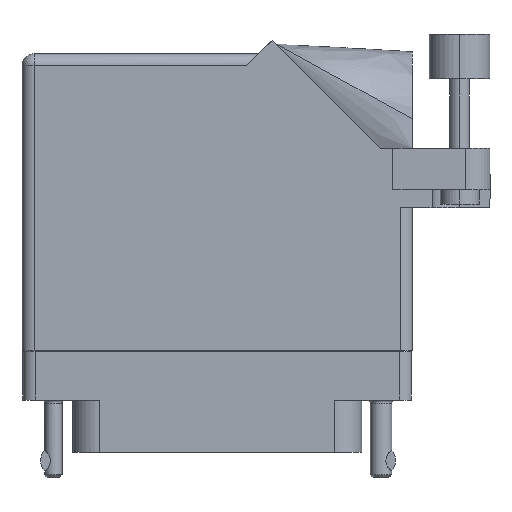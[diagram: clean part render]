
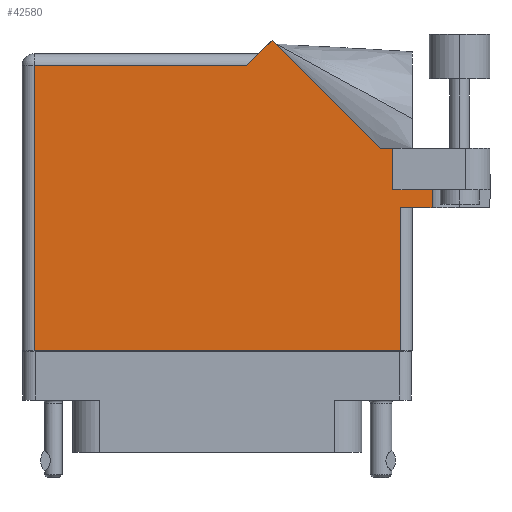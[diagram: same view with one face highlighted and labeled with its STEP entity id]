
A CAD part, front view. The second image highlights one B-rep face of the part: STEP entity #42580.
In plain terms, the highlighted face is planar.
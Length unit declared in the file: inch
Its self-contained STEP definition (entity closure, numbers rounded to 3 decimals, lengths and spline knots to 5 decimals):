
#213 = DIRECTION ( 'NONE',  ( 1., 0., 0. ) ) ;
#391 = CARTESIAN_POINT ( 'NONE',  ( -0.943, -0.1, 0.455 ) ) ;
#471 = PLANE ( 'NONE',  #19270 ) ;
#1316 = DIRECTION ( 'NONE',  ( 0., 1., 0. ) ) ;
#1674 = VECTOR ( 'NONE', #46622, 39.37008 ) ;
#4321 = CARTESIAN_POINT ( 'NONE',  ( -1.005, -0.1, 0.455 ) ) ;
#4349 = DIRECTION ( 'NONE',  ( 1., 0., 0. ) ) ;
#4591 = VERTEX_POINT ( 'NONE', #47811 ) ;
#5573 = DIRECTION ( 'NONE',  ( 1., 0., 0. ) ) ;
#5835 = CARTESIAN_POINT ( 'NONE',  ( 0.905, 0.731, 0.455 ) ) ;
#6892 = LINE ( 'NONE', #45167, #42203 ) ;
#7204 = EDGE_CURVE ( 'NONE', #48685, #36561, #42917, .T. ) ;
#8289 = CARTESIAN_POINT ( 'NONE',  ( -1.005, 1.43, 0.455 ) ) ;
#8791 = CARTESIAN_POINT ( 'NONE',  ( 0.943, 0.637, 0.455 ) ) ;
#9611 = LINE ( 'NONE', #45680, #19108 ) ;
#10578 = ORIENTED_EDGE ( 'NONE', *, *, #26713, .T. ) ;
#11178 = VECTOR ( 'NONE', #5573, 39.37008 ) ;
#11192 = VERTEX_POINT ( 'NONE', #36400 ) ;
#11431 = DIRECTION ( 'NONE',  ( -0.707, -0.707, 0. ) ) ;
#11445 = VERTEX_POINT ( 'NONE', #33540 ) ;
#11779 = CARTESIAN_POINT ( 'NONE',  ( 0.943, 0.637, 0.455 ) ) ;
#11818 = ORIENTED_EDGE ( 'NONE', *, *, #48078, .T. ) ;
#11912 = LINE ( 'NONE', #46286, #1674 ) ;
#11988 = VERTEX_POINT ( 'NONE', #46523 ) ;
#12066 = FACE_OUTER_BOUND ( 'NONE', #29427, .T. ) ;
#13126 = VECTOR ( 'NONE', #25380, 39.37008 ) ;
#14388 = LINE ( 'NONE', #33651, #33549 ) ;
#14573 = DIRECTION ( 'NONE',  ( 0., 1., 0. ) ) ;
#15288 = CARTESIAN_POINT ( 'NONE',  ( 0.83942, 0.944, 0.455 ) ) ;
#16756 = CARTESIAN_POINT ( 'NONE',  ( 1.1065, 0.637, 0.455 ) ) ;
#17214 = CARTESIAN_POINT ( 'NONE',  ( 1.005, 0.637, 0.455 ) ) ;
#17432 = LINE ( 'NONE', #8791, #44462 ) ;
#18132 = DIRECTION ( 'NONE',  ( -1., 0., 0. ) ) ;
#18425 = ORIENTED_EDGE ( 'NONE', *, *, #28230, .T. ) ;
#18794 = DIRECTION ( 'NONE',  ( -1., 0., 0. ) ) ;
#19108 = VECTOR ( 'NONE', #18794, 39.37008 ) ;
#19270 = AXIS2_PLACEMENT_3D ( 'NONE', #8289, #19598, #35013 ) ;
#19598 = DIRECTION ( 'NONE',  ( 0., 0., -1. ) ) ;
#20357 = EDGE_CURVE ( 'NONE', #48685, #4591, #14388, .T. ) ;
#20387 = LINE ( 'NONE', #48424, #45028 ) ;
#22706 = VECTOR ( 'NONE', #213, 39.37008 ) ;
#22811 = VERTEX_POINT ( 'NONE', #22966 ) ;
#22966 = CARTESIAN_POINT ( 'NONE',  ( 0.943, -0.1, 0.455 ) ) ;
#23281 = ORIENTED_EDGE ( 'NONE', *, *, #48966, .T. ) ;
#23584 = CARTESIAN_POINT ( 'NONE',  ( 0.905, 0.731, 0.455 ) ) ;
#24344 = ORIENTED_EDGE ( 'NONE', *, *, #7204, .F. ) ;
#25380 = DIRECTION ( 'NONE',  ( 0., -1., 0. ) ) ;
#26713 = EDGE_CURVE ( 'NONE', #22811, #47201, #17432, .T. ) ;
#27100 = ORIENTED_EDGE ( 'NONE', *, *, #28448, .T. ) ;
#27797 = ORIENTED_EDGE ( 'NONE', *, *, #36316, .T. ) ;
#28230 = EDGE_CURVE ( 'NONE', #11192, #11445, #37703, .T. ) ;
#28448 = EDGE_CURVE ( 'NONE', #44562, #11192, #11912, .T. ) ;
#28975 = ORIENTED_EDGE ( 'NONE', *, *, #35480, .F. ) ;
#29427 = EDGE_LOOP ( 'NONE', ( #27797, #10578, #48286, #28975, #24344, #48777, #29545, #27100, #18425, #23281, #11818 ) ) ;
#29545 = ORIENTED_EDGE ( 'NONE', *, *, #32115, .T. ) ;
#29752 = VERTEX_POINT ( 'NONE', #16756 ) ;
#30336 = EDGE_CURVE ( 'NONE', #47201, #29752, #31501, .T. ) ;
#31501 = LINE ( 'NONE', #17214, #11178 ) ;
#32115 = EDGE_CURVE ( 'NONE', #4591, #44562, #6892, .T. ) ;
#32276 = LINE ( 'NONE', #44840, #13126 ) ;
#32796 = DIRECTION ( 'NONE',  ( 0., -1., 0. ) ) ;
#33540 = CARTESIAN_POINT ( 'NONE',  ( 0.15, 1.368, 0.455 ) ) ;
#33549 = VECTOR ( 'NONE', #14573, 39.37008 ) ;
#33651 = CARTESIAN_POINT ( 'NONE',  ( 0.905, 0.731, 0.455 ) ) ;
#34340 = CARTESIAN_POINT ( 'NONE',  ( 0.212, 1.43, 0.455 ) ) ;
#35013 = DIRECTION ( 'NONE',  ( -1., 0., 0. ) ) ;
#35105 = VECTOR ( 'NONE', #4349, 39.37008 ) ;
#35480 = EDGE_CURVE ( 'NONE', #36561, #29752, #32276, .T. ) ;
#36316 = EDGE_CURVE ( 'NONE', #48310, #22811, #45548, .T. ) ;
#36400 = CARTESIAN_POINT ( 'NONE',  ( 0.28271, 1.50071, 0.455 ) ) ;
#36561 = VERTEX_POINT ( 'NONE', #36758 ) ;
#36758 = CARTESIAN_POINT ( 'NONE',  ( 1.1065, 0.731, 0.455 ) ) ;
#37703 = LINE ( 'NONE', #34340, #46119 ) ;
#42203 = VECTOR ( 'NONE', #18132, 39.37008 ) ;
#42580 = ADVANCED_FACE ( 'NONE', ( #12066 ), #471, .F. ) ;
#42917 = LINE ( 'NONE', #23584, #35105 ) ;
#44462 = VECTOR ( 'NONE', #1316, 39.37008 ) ;
#44562 = VERTEX_POINT ( 'NONE', #15288 ) ;
#44840 = CARTESIAN_POINT ( 'NONE',  ( 1.1065, 1.06177, 0.455 ) ) ;
#45028 = VECTOR ( 'NONE', #32796, 39.37008 ) ;
#45167 = CARTESIAN_POINT ( 'NONE',  ( 1.405, 0.944, 0.455 ) ) ;
#45548 = LINE ( 'NONE', #4321, #22706 ) ;
#45680 = CARTESIAN_POINT ( 'NONE',  ( -1.005, 1.368, 0.455 ) ) ;
#46119 = VECTOR ( 'NONE', #11431, 39.37008 ) ;
#46286 = CARTESIAN_POINT ( 'NONE',  ( 0.83942, 0.944, 0.455 ) ) ;
#46523 = CARTESIAN_POINT ( 'NONE',  ( -0.943, 1.368, 0.455 ) ) ;
#46622 = DIRECTION ( 'NONE',  ( -0.707, 0.707, 0. ) ) ;
#47201 = VERTEX_POINT ( 'NONE', #11779 ) ;
#47811 = CARTESIAN_POINT ( 'NONE',  ( 0.905, 0.944, 0.455 ) ) ;
#48078 = EDGE_CURVE ( 'NONE', #11988, #48310, #20387, .T. ) ;
#48286 = ORIENTED_EDGE ( 'NONE', *, *, #30336, .T. ) ;
#48310 = VERTEX_POINT ( 'NONE', #391 ) ;
#48424 = CARTESIAN_POINT ( 'NONE',  ( -0.943, -0.1, 0.455 ) ) ;
#48685 = VERTEX_POINT ( 'NONE', #5835 ) ;
#48777 = ORIENTED_EDGE ( 'NONE', *, *, #20357, .T. ) ;
#48966 = EDGE_CURVE ( 'NONE', #11445, #11988, #9611, .T. ) ;
